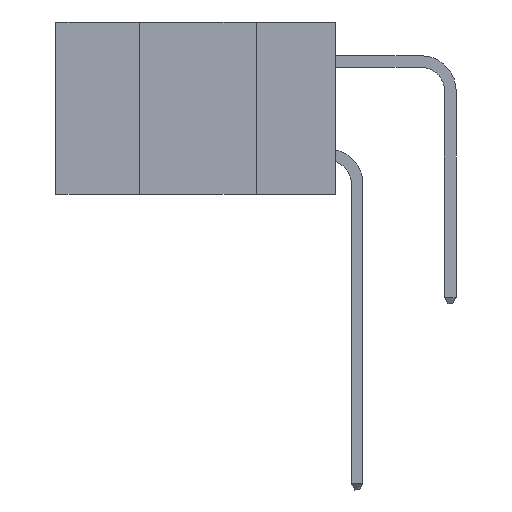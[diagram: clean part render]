
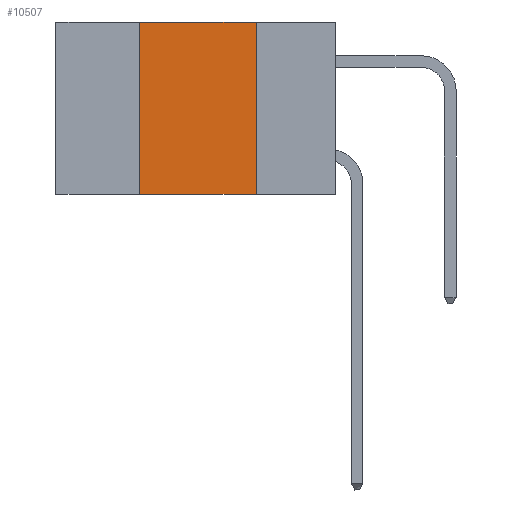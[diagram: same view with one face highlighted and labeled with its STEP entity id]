
A CAD part, left-side view. The second image highlights one B-rep face of the part: STEP entity #10507.
In plain terms, the highlighted planar face has unit normal (-1, 0, 0).
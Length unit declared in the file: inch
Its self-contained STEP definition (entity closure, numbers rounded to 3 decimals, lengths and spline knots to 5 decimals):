
#215 = PLANE ( 'NONE',  #2143 ) ;
#798 = VERTEX_POINT ( 'NONE', #7261 ) ;
#1150 = EDGE_CURVE ( 'NONE', #798, #5419, #6025, .T. ) ;
#1360 = CARTESIAN_POINT ( 'NONE',  ( 0., 0.6, 0. ) ) ;
#1364 = DIRECTION ( 'NONE',  ( 1., 0., 0. ) ) ;
#2143 = AXIS2_PLACEMENT_3D ( 'NONE', #7587, #1364, #8530 ) ;
#2238 = EDGE_LOOP ( 'NONE', ( #6616, #8130, #4389, #5365 ) ) ;
#2659 = EDGE_CURVE ( 'NONE', #4388, #9823, #11223, .T. ) ;
#2733 = EDGE_CURVE ( 'NONE', #5419, #9823, #12331, .T. ) ;
#2802 = EDGE_CURVE ( 'NONE', #4388, #798, #12081, .T. ) ;
#3166 = DIRECTION ( 'NONE',  ( 0., 0., 1. ) ) ;
#3399 = CARTESIAN_POINT ( 'NONE',  ( 0., 0.42, 0. ) ) ;
#3457 = FACE_OUTER_BOUND ( 'NONE', #2238, .T. ) ;
#3541 = VECTOR ( 'NONE', #4368, 39.37008 ) ;
#3794 = DIRECTION ( 'NONE',  ( 0., 0., -1. ) ) ;
#4156 = DIRECTION ( 'NONE',  ( 0., -1., 0. ) ) ;
#4326 = CARTESIAN_POINT ( 'NONE',  ( 0., 0.6, -0.37 ) ) ;
#4368 = DIRECTION ( 'NONE',  ( 0., -1., 0. ) ) ;
#4388 = VERTEX_POINT ( 'NONE', #8503 ) ;
#4389 = ORIENTED_EDGE ( 'NONE', *, *, #2802, .F. ) ;
#5365 = ORIENTED_EDGE ( 'NONE', *, *, #2659, .T. ) ;
#5419 = VERTEX_POINT ( 'NONE', #7406 ) ;
#5425 = CARTESIAN_POINT ( 'NONE',  ( 0., 0.17, 0. ) ) ;
#6025 = LINE ( 'NONE', #1360, #8197 ) ;
#6062 = CARTESIAN_POINT ( 'NONE',  ( 0., 0.17, -0.37 ) ) ;
#6616 = ORIENTED_EDGE ( 'NONE', *, *, #2733, .F. ) ;
#7261 = CARTESIAN_POINT ( 'NONE',  ( 0., 0.42, 0. ) ) ;
#7296 = VECTOR ( 'NONE', #3166, 39.37008 ) ;
#7406 = CARTESIAN_POINT ( 'NONE',  ( 0., 0.17, 0. ) ) ;
#7587 = CARTESIAN_POINT ( 'NONE',  ( 0., 0.6, 0. ) ) ;
#8130 = ORIENTED_EDGE ( 'NONE', *, *, #1150, .F. ) ;
#8197 = VECTOR ( 'NONE', #4156, 39.37008 ) ;
#8503 = CARTESIAN_POINT ( 'NONE',  ( 0., 0.42, -0.37 ) ) ;
#8530 = DIRECTION ( 'NONE',  ( 0., 0., -1. ) ) ;
#9823 = VERTEX_POINT ( 'NONE', #6062 ) ;
#10076 = VECTOR ( 'NONE', #3794, 39.37008 ) ;
#10507 = ADVANCED_FACE ( 'NONE', ( #3457 ), #215, .F. ) ;
#11223 = LINE ( 'NONE', #4326, #3541 ) ;
#12081 = LINE ( 'NONE', #3399, #7296 ) ;
#12331 = LINE ( 'NONE', #5425, #10076 ) ;
